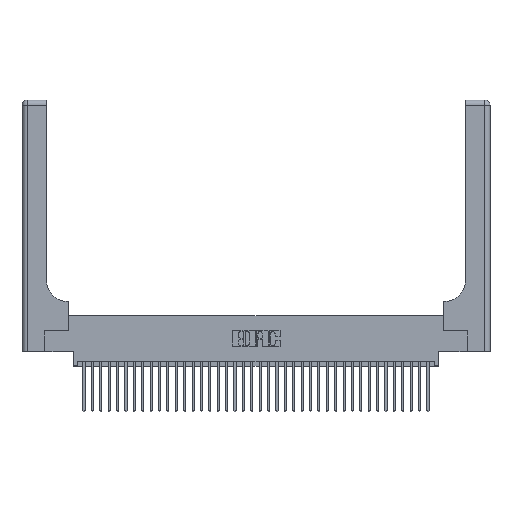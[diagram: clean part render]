
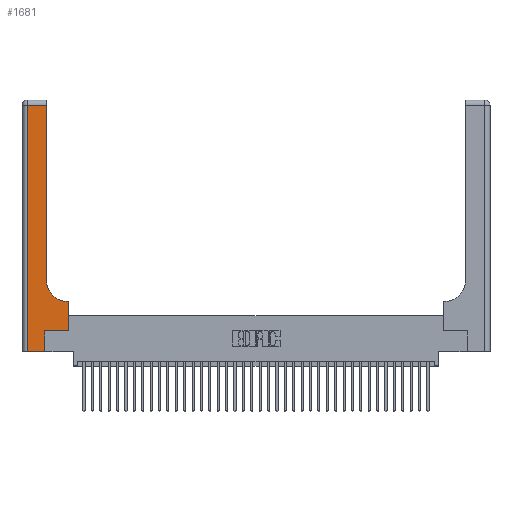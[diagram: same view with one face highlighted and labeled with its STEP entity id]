
A CAD part, top view. The second image highlights one B-rep face of the part: STEP entity #1681.
In plain terms, the highlighted planar face has unit normal (0, 0, 1).
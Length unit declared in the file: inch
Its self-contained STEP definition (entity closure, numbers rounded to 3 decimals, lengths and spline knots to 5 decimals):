
#394 = EDGE_CURVE ( 'NONE', #2394, #8382, #3719, .T. ) ;
#1040 = VERTEX_POINT ( 'NONE', #13936 ) ;
#1180 = DIRECTION ( 'NONE',  ( 0., 1., 0. ) ) ;
#1681 = ADVANCED_FACE ( 'NONE', ( #26408 ), #28427, .F. ) ;
#2265 = EDGE_LOOP ( 'NONE', ( #5381, #26078, #35903, #35715, #10821, #22819, #8450, #15244, #28509 ) ) ;
#2394 = VERTEX_POINT ( 'NONE', #12921 ) ;
#2631 = LINE ( 'NONE', #15953, #8250 ) ;
#3632 = DIRECTION ( 'NONE',  ( 1., 0., 0. ) ) ;
#3719 = LINE ( 'NONE', #9991, #24614 ) ;
#3895 = CARTESIAN_POINT ( 'NONE',  ( 0., 2.94, 0.37 ) ) ;
#4180 = VECTOR ( 'NONE', #19035, 39.37008 ) ;
#4990 = EDGE_CURVE ( 'NONE', #22549, #6185, #17625, .T. ) ;
#5381 = ORIENTED_EDGE ( 'NONE', *, *, #394, .T. ) ;
#5952 = VECTOR ( 'NONE', #10560, 39.37008 ) ;
#6185 = VERTEX_POINT ( 'NONE', #27440 ) ;
#6351 = EDGE_CURVE ( 'NONE', #12995, #7273, #2631, .T. ) ;
#6848 = CARTESIAN_POINT ( 'NONE',  ( 0.2915, 2.94, 0.37 ) ) ;
#7188 = CARTESIAN_POINT ( 'NONE',  ( 0.269, 0., 0.37 ) ) ;
#7273 = VERTEX_POINT ( 'NONE', #13584 ) ;
#8250 = VECTOR ( 'NONE', #10370, 39.37008 ) ;
#8382 = VERTEX_POINT ( 'NONE', #6848 ) ;
#8450 = ORIENTED_EDGE ( 'NONE', *, *, #20588, .T. ) ;
#9248 = VECTOR ( 'NONE', #19790, 39.37008 ) ;
#9291 = EDGE_CURVE ( 'NONE', #6185, #26797, #10854, .T. ) ;
#9715 = CARTESIAN_POINT ( 'NONE',  ( 0.269, 0., 0.37 ) ) ;
#9851 = VECTOR ( 'NONE', #34673, 39.37008 ) ;
#9991 = CARTESIAN_POINT ( 'NONE',  ( 0.2915, 3., 0.37 ) ) ;
#10370 = DIRECTION ( 'NONE',  ( -1., 0., 0. ) ) ;
#10560 = DIRECTION ( 'NONE',  ( 1., 0., 0. ) ) ;
#10655 = CARTESIAN_POINT ( 'NONE',  ( 0.06, 2.94, 0.37 ) ) ;
#10821 = ORIENTED_EDGE ( 'NONE', *, *, #27374, .T. ) ;
#10854 = LINE ( 'NONE', #19827, #9851 ) ;
#12705 = EDGE_CURVE ( 'NONE', #7273, #2394, #35937, .T. ) ;
#12921 = CARTESIAN_POINT ( 'NONE',  ( 0.2915, 0.85, 0.37 ) ) ;
#12995 = VERTEX_POINT ( 'NONE', #27321 ) ;
#13584 = CARTESIAN_POINT ( 'NONE',  ( 0.5415, 0.6, 0.37 ) ) ;
#13758 = DIRECTION ( 'NONE',  ( -1., 0., 0. ) ) ;
#13894 = LINE ( 'NONE', #31714, #5952 ) ;
#13936 = CARTESIAN_POINT ( 'NONE',  ( 0.5585, 0.25, 0.37 ) ) ;
#15244 = ORIENTED_EDGE ( 'NONE', *, *, #6351, .T. ) ;
#15582 = LINE ( 'NONE', #3895, #35924 ) ;
#15953 = CARTESIAN_POINT ( 'NONE',  ( 0.2915, 0.6, 0.37 ) ) ;
#16466 = CARTESIAN_POINT ( 'NONE',  ( 0., 3., 0.37 ) ) ;
#17486 = DIRECTION ( 'NONE',  ( 0., 1., 0. ) ) ;
#17625 = LINE ( 'NONE', #24132, #9248 ) ;
#18455 = DIRECTION ( 'NONE',  ( -1., 0., 0. ) ) ;
#19035 = DIRECTION ( 'NONE',  ( 0., 1., 0. ) ) ;
#19568 = DIRECTION ( 'NONE',  ( 0., 0., -1. ) ) ;
#19790 = DIRECTION ( 'NONE',  ( 0., -1., 0. ) ) ;
#19827 = CARTESIAN_POINT ( 'NONE',  ( 0., 0., 0.37 ) ) ;
#20588 = EDGE_CURVE ( 'NONE', #1040, #12995, #25994, .T. ) ;
#21405 = DIRECTION ( 'NONE',  ( 0., 0., -1. ) ) ;
#22081 = CARTESIAN_POINT ( 'NONE',  ( 0.5585, 0.25, 0.37 ) ) ;
#22549 = VERTEX_POINT ( 'NONE', #10655 ) ;
#22819 = ORIENTED_EDGE ( 'NONE', *, *, #29151, .T. ) ;
#23310 = AXIS2_PLACEMENT_3D ( 'NONE', #36351, #21405, #3632 ) ;
#23684 = EDGE_CURVE ( 'NONE', #8382, #22549, #15582, .T. ) ;
#24132 = CARTESIAN_POINT ( 'NONE',  ( 0.06, 3., 0.37 ) ) ;
#24614 = VECTOR ( 'NONE', #17486, 39.37008 ) ;
#25535 = LINE ( 'NONE', #7188, #4180 ) ;
#25994 = LINE ( 'NONE', #22081, #35202 ) ;
#26078 = ORIENTED_EDGE ( 'NONE', *, *, #23684, .T. ) ;
#26408 = FACE_OUTER_BOUND ( 'NONE', #2265, .T. ) ;
#26797 = VERTEX_POINT ( 'NONE', #9715 ) ;
#27321 = CARTESIAN_POINT ( 'NONE',  ( 0.5585, 0.6, 0.37 ) ) ;
#27374 = EDGE_CURVE ( 'NONE', #26797, #34834, #25535, .T. ) ;
#27440 = CARTESIAN_POINT ( 'NONE',  ( 0.06, 0., 0.37 ) ) ;
#28427 = PLANE ( 'NONE',  #35777 ) ;
#28509 = ORIENTED_EDGE ( 'NONE', *, *, #12705, .T. ) ;
#29151 = EDGE_CURVE ( 'NONE', #34834, #1040, #13894, .T. ) ;
#31714 = CARTESIAN_POINT ( 'NONE',  ( 0.269, 0.25, 0.37 ) ) ;
#34673 = DIRECTION ( 'NONE',  ( 1., 0., 0. ) ) ;
#34834 = VERTEX_POINT ( 'NONE', #35511 ) ;
#35202 = VECTOR ( 'NONE', #1180, 39.37008 ) ;
#35511 = CARTESIAN_POINT ( 'NONE',  ( 0.269, 0.25, 0.37 ) ) ;
#35715 = ORIENTED_EDGE ( 'NONE', *, *, #9291, .T. ) ;
#35777 = AXIS2_PLACEMENT_3D ( 'NONE', #16466, #19568, #13758 ) ;
#35903 = ORIENTED_EDGE ( 'NONE', *, *, #4990, .T. ) ;
#35924 = VECTOR ( 'NONE', #18455, 39.37008 ) ;
#35937 = CIRCLE ( 'NONE', #23310, 0.25 ) ;
#36351 = CARTESIAN_POINT ( 'NONE',  ( 0.5415, 0.85, 0.37 ) ) ;
